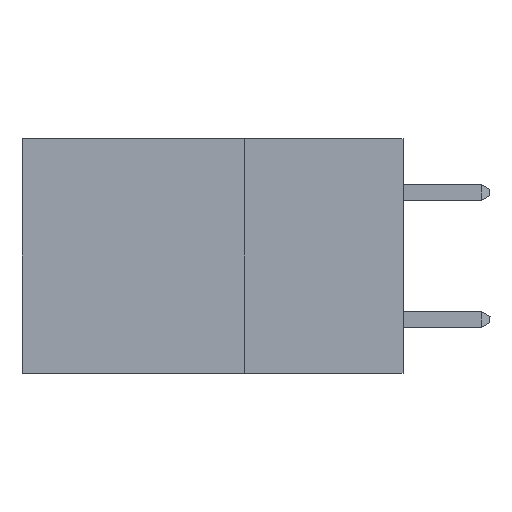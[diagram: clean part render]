
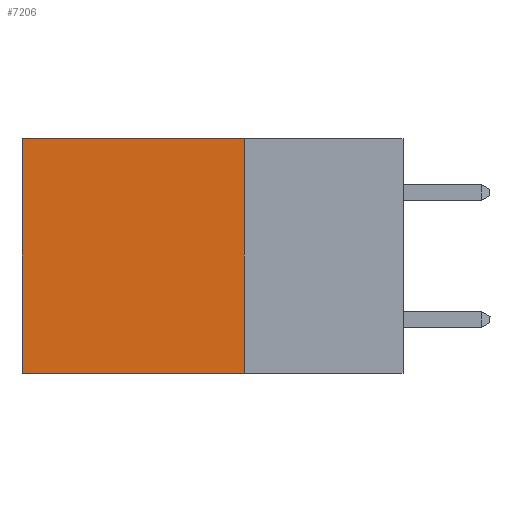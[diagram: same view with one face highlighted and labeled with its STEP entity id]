
A CAD part, left-side view. The second image highlights one B-rep face of the part: STEP entity #7206.
In plain terms, the highlighted planar face has unit normal (-1, 0, 0).
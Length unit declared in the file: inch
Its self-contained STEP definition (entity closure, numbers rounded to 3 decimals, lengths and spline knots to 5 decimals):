
#739 = VERTEX_POINT ( 'NONE', #7761 ) ;
#747 = DIRECTION ( 'NONE',  ( 0., 1., 0. ) ) ;
#1288 = VECTOR ( 'NONE', #25449, 39.37008 ) ;
#2190 = LINE ( 'NONE', #20571, #24401 ) ;
#3513 = ORIENTED_EDGE ( 'NONE', *, *, #18554, .T. ) ;
#3572 = CARTESIAN_POINT ( 'NONE',  ( 0.2875, 0.25, -0.37 ) ) ;
#3685 = EDGE_CURVE ( 'NONE', #10052, #13315, #14336, .T. ) ;
#4783 = EDGE_CURVE ( 'NONE', #739, #15432, #14403, .T. ) ;
#5949 = ORIENTED_EDGE ( 'NONE', *, *, #3685, .F. ) ;
#7206 = ADVANCED_FACE ( 'NONE', ( #8759 ), #15609, .F. ) ;
#7761 = CARTESIAN_POINT ( 'NONE',  ( 0.2875, 0.6, 0. ) ) ;
#8324 = EDGE_LOOP ( 'NONE', ( #11123, #18434, #5949, #3513 ) ) ;
#8759 = FACE_OUTER_BOUND ( 'NONE', #8324, .T. ) ;
#10052 = VERTEX_POINT ( 'NONE', #17356 ) ;
#11123 = ORIENTED_EDGE ( 'NONE', *, *, #4783, .T. ) ;
#11860 = CARTESIAN_POINT ( 'NONE',  ( 0.2875, 0.6, 0. ) ) ;
#12698 = VECTOR ( 'NONE', #21209, 39.37008 ) ;
#13315 = VERTEX_POINT ( 'NONE', #3572 ) ;
#13449 = EDGE_CURVE ( 'NONE', #13315, #15432, #2190, .T. ) ;
#14336 = LINE ( 'NONE', #23145, #12698 ) ;
#14403 = LINE ( 'NONE', #11860, #1288 ) ;
#15432 = VERTEX_POINT ( 'NONE', #28745 ) ;
#15474 = DIRECTION ( 'NONE',  ( 0., 0., -1. ) ) ;
#15609 = PLANE ( 'NONE',  #16098 ) ;
#15983 = CARTESIAN_POINT ( 'NONE',  ( 0.2875, 0.25, 0. ) ) ;
#16098 = AXIS2_PLACEMENT_3D ( 'NONE', #29062, #17711, #15474 ) ;
#17356 = CARTESIAN_POINT ( 'NONE',  ( 0.2875, 0.25, 0. ) ) ;
#17711 = DIRECTION ( 'NONE',  ( 1., 0., 0. ) ) ;
#18029 = DIRECTION ( 'NONE',  ( 0., 1., 0. ) ) ;
#18434 = ORIENTED_EDGE ( 'NONE', *, *, #13449, .F. ) ;
#18554 = EDGE_CURVE ( 'NONE', #10052, #739, #21220, .T. ) ;
#20571 = CARTESIAN_POINT ( 'NONE',  ( 0.2875, 0.25, -0.37 ) ) ;
#21209 = DIRECTION ( 'NONE',  ( 0., 0., -1. ) ) ;
#21220 = LINE ( 'NONE', #15983, #22204 ) ;
#22204 = VECTOR ( 'NONE', #747, 39.37008 ) ;
#23145 = CARTESIAN_POINT ( 'NONE',  ( 0.2875, 0.25, 0. ) ) ;
#24401 = VECTOR ( 'NONE', #18029, 39.37008 ) ;
#25449 = DIRECTION ( 'NONE',  ( 0., 0., -1. ) ) ;
#28745 = CARTESIAN_POINT ( 'NONE',  ( 0.2875, 0.6, -0.37 ) ) ;
#29062 = CARTESIAN_POINT ( 'NONE',  ( 0.2875, 0.25, 0. ) ) ;
